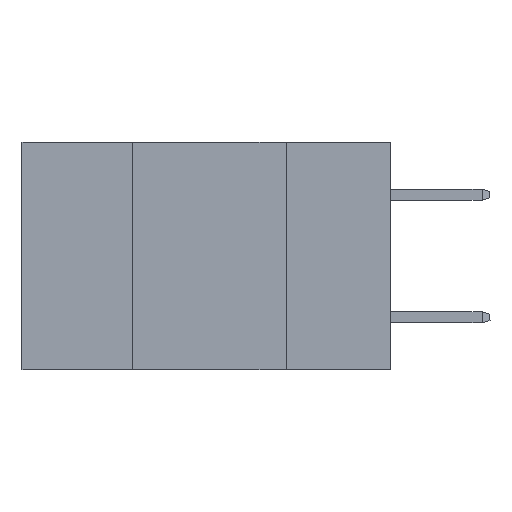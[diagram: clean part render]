
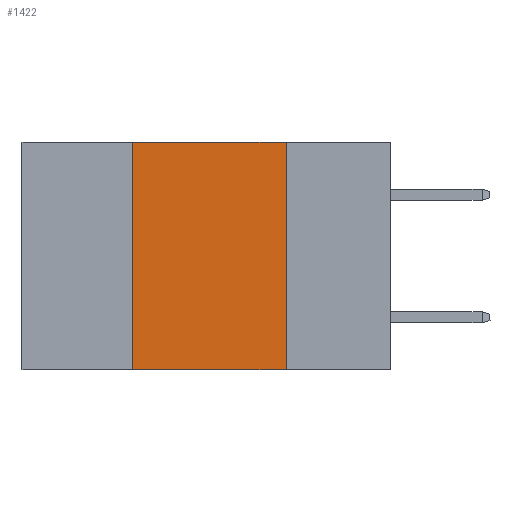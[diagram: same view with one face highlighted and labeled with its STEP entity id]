
A CAD part, left-side view. The second image highlights one B-rep face of the part: STEP entity #1422.
In plain terms, the highlighted planar face has unit normal (-1, 0, 0).
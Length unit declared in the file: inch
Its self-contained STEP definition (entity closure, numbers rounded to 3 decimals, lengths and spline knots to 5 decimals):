
#51 = VERTEX_POINT ( 'NONE', #503 ) ;
#503 = CARTESIAN_POINT ( 'NONE',  ( 0., 0.42, 0. ) ) ;
#653 = CARTESIAN_POINT ( 'NONE',  ( 0., 0.6, -0.37 ) ) ;
#711 = DIRECTION ( 'NONE',  ( 0., -1., 0. ) ) ;
#1422 = ADVANCED_FACE ( 'NONE', ( #5149 ), #2170, .F. ) ;
#1509 = CARTESIAN_POINT ( 'NONE',  ( 0., 0.17, 0. ) ) ;
#1543 = DIRECTION ( 'NONE',  ( 1., 0., 0. ) ) ;
#1641 = EDGE_CURVE ( 'NONE', #51, #2328, #8216, .T. ) ;
#1739 = DIRECTION ( 'NONE',  ( 0., -1., 0. ) ) ;
#2170 = PLANE ( 'NONE',  #7351 ) ;
#2328 = VERTEX_POINT ( 'NONE', #8950 ) ;
#2602 = ORIENTED_EDGE ( 'NONE', *, *, #6660, .F. ) ;
#2944 = DIRECTION ( 'NONE',  ( 0., 0., -1. ) ) ;
#3069 = CARTESIAN_POINT ( 'NONE',  ( 0., 0.42, -0.37 ) ) ;
#3652 = EDGE_CURVE ( 'NONE', #8309, #7053, #8093, .T. ) ;
#4299 = VECTOR ( 'NONE', #1739, 39.37008 ) ;
#4317 = DIRECTION ( 'NONE',  ( 0., 0., 1. ) ) ;
#4440 = LINE ( 'NONE', #1509, #6846 ) ;
#4546 = VECTOR ( 'NONE', #4317, 39.37008 ) ;
#4622 = CARTESIAN_POINT ( 'NONE',  ( 0., 0.6, 0. ) ) ;
#4843 = ORIENTED_EDGE ( 'NONE', *, *, #8083, .F. ) ;
#5149 = FACE_OUTER_BOUND ( 'NONE', #8297, .T. ) ;
#5218 = ORIENTED_EDGE ( 'NONE', *, *, #3652, .T. ) ;
#5842 = CARTESIAN_POINT ( 'NONE',  ( 0., 0.17, -0.37 ) ) ;
#6398 = LINE ( 'NONE', #8636, #4546 ) ;
#6556 = CARTESIAN_POINT ( 'NONE',  ( 0., 0.6, 0. ) ) ;
#6653 = DIRECTION ( 'NONE',  ( 0., 0., -1. ) ) ;
#6660 = EDGE_CURVE ( 'NONE', #8309, #51, #6398, .T. ) ;
#6846 = VECTOR ( 'NONE', #6653, 39.37008 ) ;
#7053 = VERTEX_POINT ( 'NONE', #5842 ) ;
#7351 = AXIS2_PLACEMENT_3D ( 'NONE', #6556, #1543, #2944 ) ;
#7689 = ORIENTED_EDGE ( 'NONE', *, *, #1641, .F. ) ;
#7946 = VECTOR ( 'NONE', #711, 39.37008 ) ;
#8083 = EDGE_CURVE ( 'NONE', #2328, #7053, #4440, .T. ) ;
#8093 = LINE ( 'NONE', #653, #7946 ) ;
#8216 = LINE ( 'NONE', #4622, #4299 ) ;
#8297 = EDGE_LOOP ( 'NONE', ( #4843, #7689, #2602, #5218 ) ) ;
#8309 = VERTEX_POINT ( 'NONE', #3069 ) ;
#8636 = CARTESIAN_POINT ( 'NONE',  ( 0., 0.42, 0. ) ) ;
#8950 = CARTESIAN_POINT ( 'NONE',  ( 0., 0.17, 0. ) ) ;
